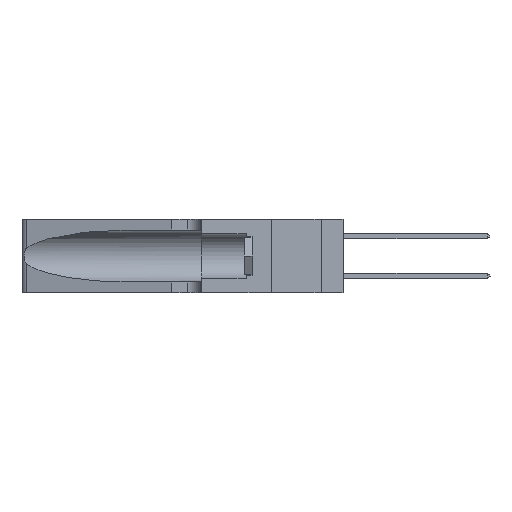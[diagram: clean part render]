
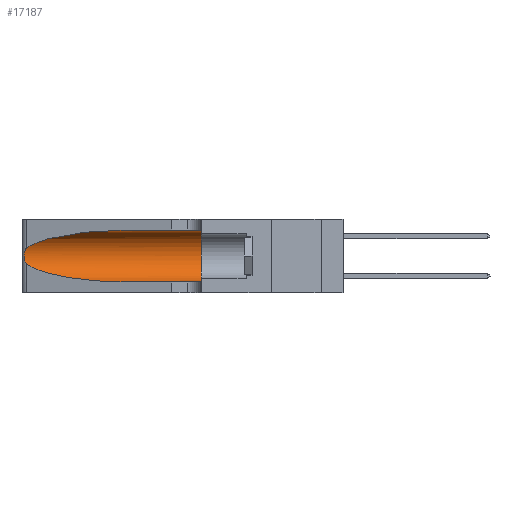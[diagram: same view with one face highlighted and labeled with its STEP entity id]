
A CAD part, left-side view. The second image highlights one B-rep face of the part: STEP entity #17187.
In plain terms, the highlighted cylindrical face has radius 3.308 mm (diameter 6.617 mm), a partial arc.
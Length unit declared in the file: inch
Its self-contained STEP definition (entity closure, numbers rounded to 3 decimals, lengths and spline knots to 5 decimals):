
#178 = CARTESIAN_POINT ( 'NONE',  ( 0.25487, 1.22718, 0.22369 ) ) ;
#235 = ORIENTED_EDGE ( 'NONE', *, *, #18040, .F. ) ;
#355 = EDGE_CURVE ( 'NONE', #2852, #7709, #25569, .T. ) ;
#1177 = DIRECTION ( 'NONE',  ( 0., 0., 1. ) ) ;
#1339 = LINE ( 'NONE', #12972, #27510 ) ;
#2345 = CARTESIAN_POINT ( 'NONE',  ( 0.25555, 1.22993, 0.14849 ) ) ;
#2712 = CARTESIAN_POINT ( 'NONE',  ( 0.18966, 0.96281, 0.31525 ) ) ;
#2852 = VERTEX_POINT ( 'NONE', #15397 ) ;
#3416 = DIRECTION ( 'NONE',  ( 0., -1., 0. ) ) ;
#3585 = CARTESIAN_POINT ( 'NONE',  ( 0.25487, 1.22718, 0.14631 ) ) ;
#4013 = LINE ( 'NONE', #22695, #8027 ) ;
#4309 = CARTESIAN_POINT ( 'NONE',  ( 0.1305, 0.72297, 0.05475 ) ) ;
#4434 = VERTEX_POINT ( 'NONE', #33697 ) ;
#4979 = CARTESIAN_POINT ( 'NONE',  ( 0.25487, 1.22718, 0.14631 ) ) ;
#6081 = ORIENTED_EDGE ( 'NONE', *, *, #14239, .T. ) ;
#6593 = ORIENTED_EDGE ( 'NONE', *, *, #355, .T. ) ;
#6668 = CARTESIAN_POINT ( 'NONE',  ( 0.18966, 0.96281, 0.05475 ) ) ;
#7709 = VERTEX_POINT ( 'NONE', #19948 ) ;
#8005 = CARTESIAN_POINT ( 'NONE',  ( 0.25639, 1.23186, 0.15144 ) ) ;
#8027 = VECTOR ( 'NONE', #3416, 39.37008 ) ;
#8057 = CARTESIAN_POINT ( 'NONE',  ( 0.1305, 0.72297, 0.31525 ) ) ;
#9201 = CARTESIAN_POINT ( 'NONE',  ( 0.1305, 0.35, 0.185 ) ) ;
#10263 = EDGE_CURVE ( 'NONE', #28398, #4434, #4013, .T. ) ;
#10561 = CARTESIAN_POINT ( 'NONE',  ( 0.26018, 1.23835, 0.19895 ) ) ;
#10601 = ORIENTED_EDGE ( 'NONE', *, *, #10263, .F. ) ;
#11525 = ORIENTED_EDGE ( 'NONE', *, *, #23142, .T. ) ;
#11888 = CARTESIAN_POINT ( 'NONE',  ( 0.1305, 0.35, 0.05475 ) ) ;
#12818 = CARTESIAN_POINT ( 'NONE',  ( 0.25487, 1.22718, 0.22369 ) ) ;
#12878 = CARTESIAN_POINT ( 'NONE',  ( 0.26075, 1.23896, 0.19203 ) ) ;
#12972 = CARTESIAN_POINT ( 'NONE',  ( 0.1305, 1.61858, 0.05475 ) ) ;
#13020 = CARTESIAN_POINT ( 'NONE',  ( 0.25639, 1.23184, 0.21858 ) ) ;
#13085 = CARTESIAN_POINT ( 'NONE',  ( 0.26075, 1.23896, 0.178 ) ) ;
#14239 = EDGE_CURVE ( 'NONE', #7709, #30229, #20972, .T. ) ;
#15397 = CARTESIAN_POINT ( 'NONE',  ( 0.25487, 1.22718, 0.22369 ) ) ;
#15401 = CARTESIAN_POINT ( 'NONE',  ( 0.25555, 1.22994, 0.2215 ) ) ;
#15788 = CARTESIAN_POINT ( 'NONE',  ( 0.25789, 1.23486, 0.15765 ) ) ;
#15836 = CARTESIAN_POINT ( 'NONE',  ( 0.1305, 0.72297, 0.31525 ) ) ;
#16135 = CARTESIAN_POINT ( 'NONE',  ( 0.25854, 1.2359, 0.20912 ) ) ;
#16943 =( BOUNDED_CURVE ( )  B_SPLINE_CURVE ( 3, ( #15836, #2712, #28532, #178 ),
 .UNSPECIFIED., .F., .F. ) 
 B_SPLINE_CURVE_WITH_KNOTS ( ( 4, 4 ),
 ( 1.5708, 2.84003 ),
 .UNSPECIFIED. ) 
 CURVE ( )  GEOMETRIC_REPRESENTATION_ITEM ( )  RATIONAL_B_SPLINE_CURVE ( ( 1., 0.87, 0.87, 1. ) ) 
 REPRESENTATION_ITEM ( '' )  );
#17187 = ADVANCED_FACE ( 'NONE', ( #29431 ), #32303, .F. ) ;
#18040 = EDGE_CURVE ( 'NONE', #4434, #30686, #30663, .T. ) ;
#19948 = CARTESIAN_POINT ( 'NONE',  ( 0.25487, 1.22718, 0.14631 ) ) ;
#20854 = CARTESIAN_POINT ( 'NONE',  ( 0.1305, 0.72297, 0.05475 ) ) ;
#20972 =( BOUNDED_CURVE ( )  B_SPLINE_CURVE ( 3, ( #3585, #32355, #6668, #4309 ),
 .UNSPECIFIED., .F., .F. ) 
 B_SPLINE_CURVE_WITH_KNOTS ( ( 4, 4 ),
 ( 3.44316, 4.71239 ),
 .UNSPECIFIED. ) 
 CURVE ( )  GEOMETRIC_REPRESENTATION_ITEM ( )  RATIONAL_B_SPLINE_CURVE ( ( 1., 0.87, 0.87, 1. ) ) 
 REPRESENTATION_ITEM ( '' )  );
#22120 = CARTESIAN_POINT ( 'NONE',  ( 0.1305, 1.61858, 0.185 ) ) ;
#22695 = CARTESIAN_POINT ( 'NONE',  ( 0.1305, 1.61858, 0.31525 ) ) ;
#22731 = AXIS2_PLACEMENT_3D ( 'NONE', #22120, #27530, #30051 ) ;
#23142 = EDGE_CURVE ( 'NONE', #28398, #2852, #16943, .T. ) ;
#25077 = AXIS2_PLACEMENT_3D ( 'NONE', #9201, #32492, #1177 ) ;
#25569 = B_SPLINE_CURVE_WITH_KNOTS ( 'NONE', 3,
 ( #12818, #15401, #13020, #28522, #16135, #10561, #12878, #13085, #31425, #31119, #15788, #8005, #2345, #4979 ),
 .UNSPECIFIED., .F., .F.,
 ( 4, 2, 2, 2, 2, 2, 4 ),
 ( 0., 0.00027, 0.00053, 0.00107, 0.0016, 0.00187, 0.00214 ),
 .UNSPECIFIED. ) ;
#27510 = VECTOR ( 'NONE', #28361, 39.37008 ) ;
#27521 = EDGE_LOOP ( 'NONE', ( #11525, #6593, #6081, #32294, #235, #10601 ) ) ;
#27530 = DIRECTION ( 'NONE',  ( 0., -1., 0. ) ) ;
#27667 = EDGE_CURVE ( 'NONE', #30229, #30686, #1339, .T. ) ;
#28361 = DIRECTION ( 'NONE',  ( 0., -1., 0. ) ) ;
#28398 = VERTEX_POINT ( 'NONE', #8057 ) ;
#28522 = CARTESIAN_POINT ( 'NONE',  ( 0.25787, 1.23484, 0.2124 ) ) ;
#28532 = CARTESIAN_POINT ( 'NONE',  ( 0.2373, 1.15595, 0.28018 ) ) ;
#29431 = FACE_OUTER_BOUND ( 'NONE', #27521, .T. ) ;
#30051 = DIRECTION ( 'NONE',  ( 0., 0., -1. ) ) ;
#30229 = VERTEX_POINT ( 'NONE', #20854 ) ;
#30663 = CIRCLE ( 'NONE', #25077, 0.13025 ) ;
#30686 = VERTEX_POINT ( 'NONE', #11888 ) ;
#31119 = CARTESIAN_POINT ( 'NONE',  ( 0.25856, 1.23593, 0.16098 ) ) ;
#31425 = CARTESIAN_POINT ( 'NONE',  ( 0.26017, 1.23833, 0.17102 ) ) ;
#32294 = ORIENTED_EDGE ( 'NONE', *, *, #27667, .T. ) ;
#32303 = CYLINDRICAL_SURFACE ( 'NONE', #22731, 0.13025 ) ;
#32355 = CARTESIAN_POINT ( 'NONE',  ( 0.2373, 1.15595, 0.08982 ) ) ;
#32492 = DIRECTION ( 'NONE',  ( 0., 1., 0. ) ) ;
#33697 = CARTESIAN_POINT ( 'NONE',  ( 0.1305, 0.35, 0.31525 ) ) ;
